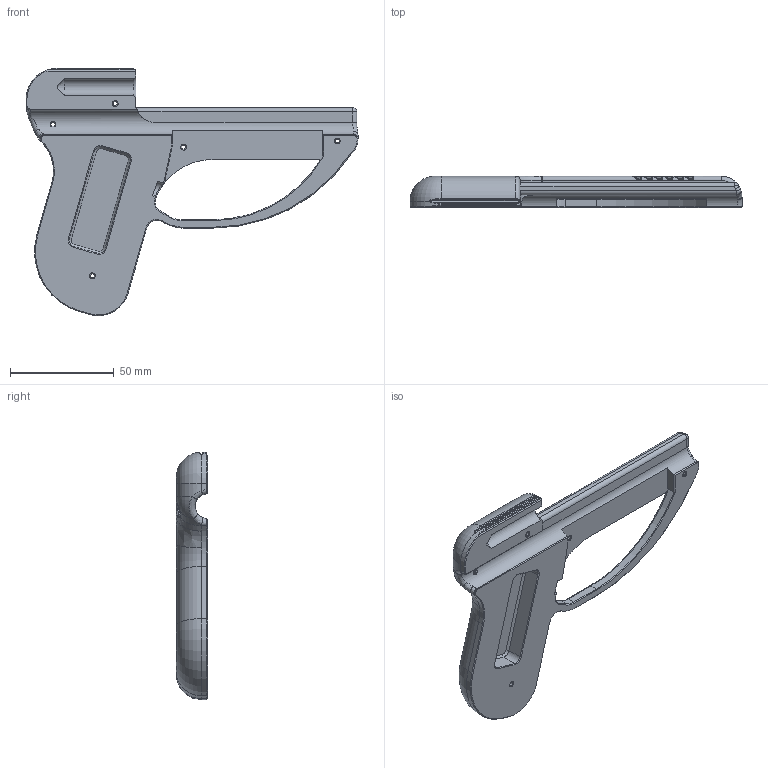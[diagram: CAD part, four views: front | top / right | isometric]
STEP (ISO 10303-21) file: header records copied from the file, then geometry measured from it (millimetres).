
FILE_DESCRIPTION(('FreeCAD Model'),'2;1');
FILE_NAME('Open CASCADE Shape Model','2022-12-07T11:23:36',('Author'),( ''),'Open CASCADE STEP processor 7.6','FreeCAD','Unknown');
FILE_SCHEMA(('AUTOMOTIVE_DESIGN { 1 0 10303 214 1 1 1 1 }'));
Length unit declared in the file: millimetre
Products named in the file (1): Frame-Left
Bounding box: 160 x 15 x 119.19 mm (x, y, z)
Volume: 88396.9 mm3; surface area: 25898.2 mm2
Topology: 1 solids, 1 shells, 685 faces, 1840 edges, 1155 vertices
Faces by surface type: plane 388, bspline 169, cylinder 75, cone 33, torus 16, revolution 4
Full cylindrical faces by diameter (mm): 2 x5
Entity records: 67032 total; most frequent: CARTESIAN_POINT 34461, DIRECTION 4766, ORIENTED_EDGE 3674, PCURVE 3674, DEFINITIONAL_REPRESENTATION 3674, LINE 3326, VECTOR 3326, EDGE_CURVE 1837
